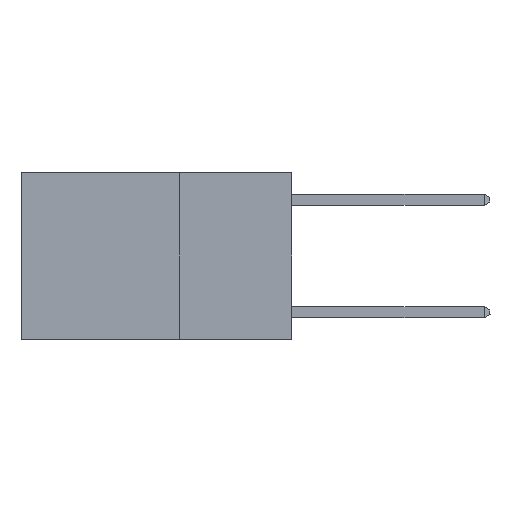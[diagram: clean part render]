
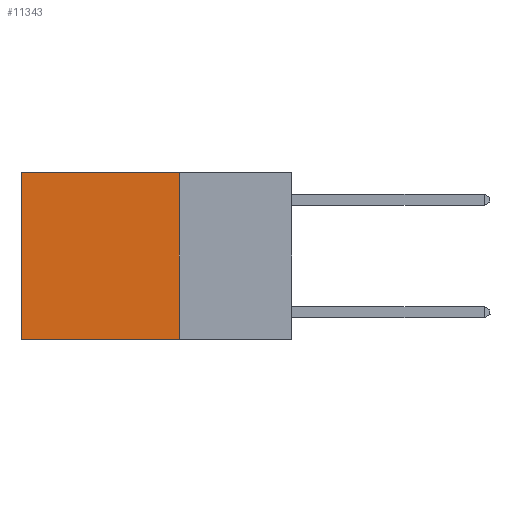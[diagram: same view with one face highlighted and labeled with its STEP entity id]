
A CAD part, left-side view. The second image highlights one B-rep face of the part: STEP entity #11343.
In plain terms, the highlighted planar face has unit normal (-1, 0, 0).
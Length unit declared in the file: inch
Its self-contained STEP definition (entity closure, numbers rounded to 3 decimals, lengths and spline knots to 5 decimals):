
#608 = CARTESIAN_POINT ( 'NONE',  ( 0.2625, 0.6, -0.37 ) ) ;
#1463 = VECTOR ( 'NONE', #7967, 39.37008 ) ;
#1500 = ORIENTED_EDGE ( 'NONE', *, *, #20005, .F. ) ;
#2836 = VERTEX_POINT ( 'NONE', #608 ) ;
#3002 = CARTESIAN_POINT ( 'NONE',  ( 0.2625, 0.25, 0. ) ) ;
#3530 = CARTESIAN_POINT ( 'NONE',  ( 0.2625, 0.6, 0. ) ) ;
#3719 = LINE ( 'NONE', #22519, #12592 ) ;
#3990 = PLANE ( 'NONE',  #8325 ) ;
#5662 = EDGE_CURVE ( 'NONE', #15052, #6869, #19147, .T. ) ;
#5884 = CARTESIAN_POINT ( 'NONE',  ( 0.2625, 0.25, 0. ) ) ;
#6815 = VERTEX_POINT ( 'NONE', #7240 ) ;
#6869 = VERTEX_POINT ( 'NONE', #3530 ) ;
#7228 = DIRECTION ( 'NONE',  ( 0., 0., -1. ) ) ;
#7240 = CARTESIAN_POINT ( 'NONE',  ( 0.2625, 0.25, -0.37 ) ) ;
#7653 = EDGE_CURVE ( 'NONE', #6815, #2836, #3719, .T. ) ;
#7853 = DIRECTION ( 'NONE',  ( 1., 0., 0. ) ) ;
#7967 = DIRECTION ( 'NONE',  ( 0., 0., -1. ) ) ;
#8191 = VECTOR ( 'NONE', #7228, 39.37008 ) ;
#8325 = AXIS2_PLACEMENT_3D ( 'NONE', #5884, #7853, #20753 ) ;
#9333 = DIRECTION ( 'NONE',  ( 0., 1., 0. ) ) ;
#11343 = ADVANCED_FACE ( 'NONE', ( #18524 ), #3990, .F. ) ;
#12592 = VECTOR ( 'NONE', #17178, 39.37008 ) ;
#14800 = VECTOR ( 'NONE', #9333, 39.37008 ) ;
#15052 = VERTEX_POINT ( 'NONE', #3002 ) ;
#15755 = EDGE_LOOP ( 'NONE', ( #18380, #19577, #1500, #19309 ) ) ;
#17178 = DIRECTION ( 'NONE',  ( 0., 1., 0. ) ) ;
#18380 = ORIENTED_EDGE ( 'NONE', *, *, #23869, .T. ) ;
#18524 = FACE_OUTER_BOUND ( 'NONE', #15755, .T. ) ;
#19147 = LINE ( 'NONE', #20369, #14800 ) ;
#19309 = ORIENTED_EDGE ( 'NONE', *, *, #5662, .T. ) ;
#19577 = ORIENTED_EDGE ( 'NONE', *, *, #7653, .F. ) ;
#20005 = EDGE_CURVE ( 'NONE', #15052, #6815, #21850, .T. ) ;
#20181 = CARTESIAN_POINT ( 'NONE',  ( 0.2625, 0.6, 0. ) ) ;
#20369 = CARTESIAN_POINT ( 'NONE',  ( 0.2625, 0.25, 0. ) ) ;
#20753 = DIRECTION ( 'NONE',  ( 0., 0., -1. ) ) ;
#20866 = CARTESIAN_POINT ( 'NONE',  ( 0.2625, 0.25, 0. ) ) ;
#21850 = LINE ( 'NONE', #20866, #1463 ) ;
#22519 = CARTESIAN_POINT ( 'NONE',  ( 0.2625, 0.25, -0.37 ) ) ;
#22752 = LINE ( 'NONE', #20181, #8191 ) ;
#23869 = EDGE_CURVE ( 'NONE', #6869, #2836, #22752, .T. ) ;
